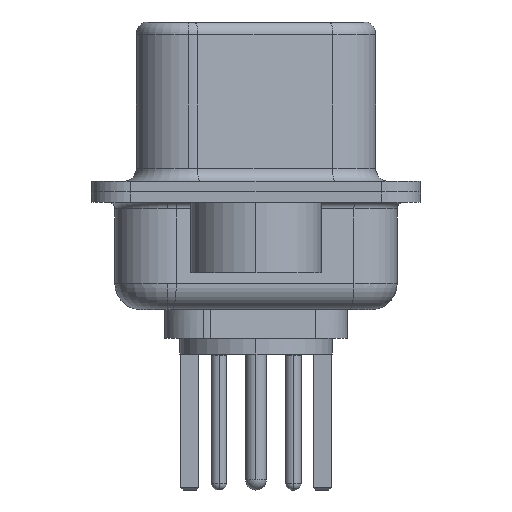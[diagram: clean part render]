
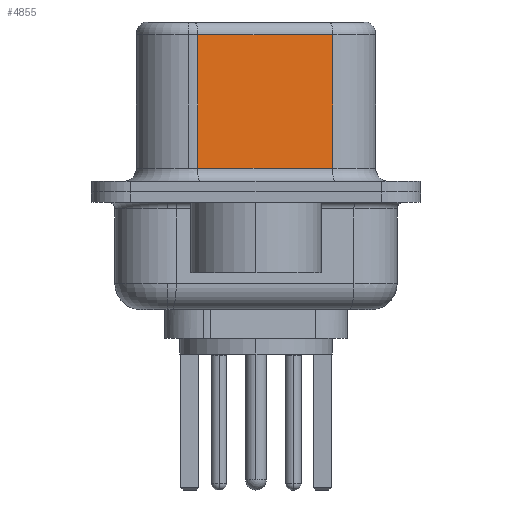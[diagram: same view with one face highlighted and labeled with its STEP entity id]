
A CAD part, left-side view. The second image highlights one B-rep face of the part: STEP entity #4855.
In plain terms, the highlighted planar face has unit normal (-0.985, -0.174, 0).
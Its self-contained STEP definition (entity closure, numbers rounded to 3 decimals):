
#259 = LINE ( 'NONE', #13141, #2359 ) ;
#2359 = VECTOR ( 'NONE', #7261, 1000. ) ;
#3058 = ORIENTED_EDGE ( 'NONE', *, *, #15536, .T. ) ;
#3841 = LINE ( 'NONE', #15459, #23530 ) ;
#4855 = ADVANCED_FACE ( 'NONE', ( #12871 ), #5021, .F. ) ;
#5021 = PLANE ( 'NONE',  #14054 ) ;
#5121 = VERTEX_POINT ( 'NONE', #13696 ) ;
#5712 = VECTOR ( 'NONE', #8276, 1000. ) ;
#7233 = VECTOR ( 'NONE', #24519, 1000. ) ;
#7261 = DIRECTION ( 'NONE',  ( -0.174, 0.985, 0. ) ) ;
#7824 = DIRECTION ( 'NONE',  ( 0.174, -0.985, 0. ) ) ;
#7936 = EDGE_LOOP ( 'NONE', ( #23809, #3058, #20849, #22512 ) ) ;
#8276 = DIRECTION ( 'NONE',  ( 0., 0., -1. ) ) ;
#10456 = EDGE_CURVE ( 'NONE', #19003, #5121, #15366, .T. ) ;
#10694 = DIRECTION ( 'NONE',  ( 0.985, 0.174, 0. ) ) ;
#10852 = DIRECTION ( 'NONE',  ( -0.174, 0.985, 0. ) ) ;
#11996 = LINE ( 'NONE', #17692, #5712 ) ;
#12057 = EDGE_CURVE ( 'NONE', #19464, #22605, #11996, .T. ) ;
#12871 = FACE_OUTER_BOUND ( 'NONE', #7936, .T. ) ;
#13141 = CARTESIAN_POINT ( 'NONE',  ( 4.585, -2.927, 6.02 ) ) ;
#13696 = CARTESIAN_POINT ( 'NONE',  ( 3.675, 2.233, 0.9 ) ) ;
#14054 = AXIS2_PLACEMENT_3D ( 'NONE', #16611, #10694, #10852 ) ;
#15366 = LINE ( 'NONE', #16750, #7233 ) ;
#15459 = CARTESIAN_POINT ( 'NONE',  ( 4.585, -2.927, 0.9 ) ) ;
#15536 = EDGE_CURVE ( 'NONE', #19464, #19003, #259, .T. ) ;
#16184 = EDGE_CURVE ( 'NONE', #5121, #22605, #3841, .T. ) ;
#16575 = CARTESIAN_POINT ( 'NONE',  ( 4.585, -2.927, 6.02 ) ) ;
#16611 = CARTESIAN_POINT ( 'NONE',  ( 4.585, -2.927, 6.52 ) ) ;
#16750 = CARTESIAN_POINT ( 'NONE',  ( 3.675, 2.233, 6.52 ) ) ;
#17692 = CARTESIAN_POINT ( 'NONE',  ( 4.585, -2.927, 6.52 ) ) ;
#19003 = VERTEX_POINT ( 'NONE', #21678 ) ;
#19464 = VERTEX_POINT ( 'NONE', #16575 ) ;
#20849 = ORIENTED_EDGE ( 'NONE', *, *, #10456, .T. ) ;
#21678 = CARTESIAN_POINT ( 'NONE',  ( 3.675, 2.233, 6.02 ) ) ;
#22512 = ORIENTED_EDGE ( 'NONE', *, *, #16184, .T. ) ;
#22605 = VERTEX_POINT ( 'NONE', #24218 ) ;
#23530 = VECTOR ( 'NONE', #7824, 1000. ) ;
#23809 = ORIENTED_EDGE ( 'NONE', *, *, #12057, .F. ) ;
#24218 = CARTESIAN_POINT ( 'NONE',  ( 4.585, -2.927, 0.9 ) ) ;
#24519 = DIRECTION ( 'NONE',  ( 0., 0., -1. ) ) ;
